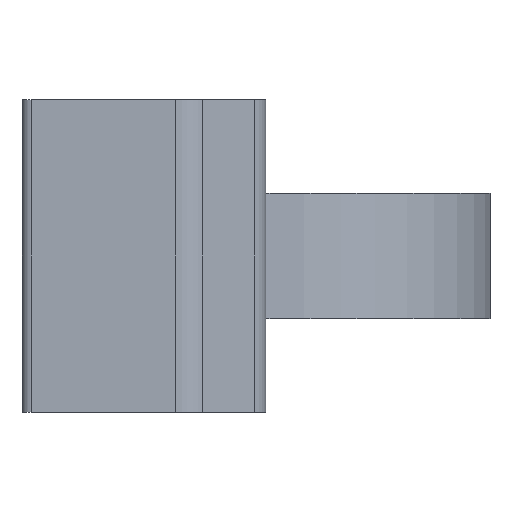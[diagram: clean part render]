
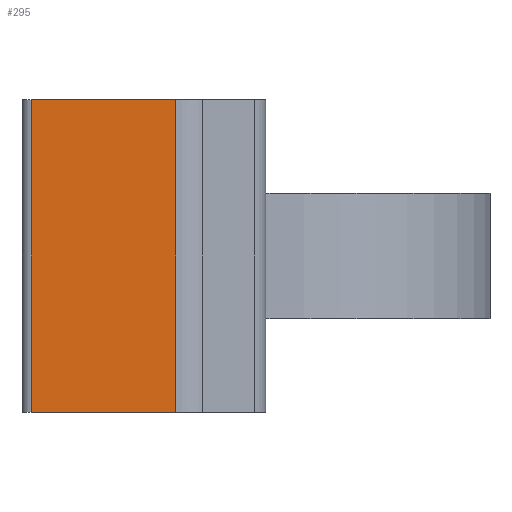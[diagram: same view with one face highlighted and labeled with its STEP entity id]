
A CAD part, front view. The second image highlights one B-rep face of the part: STEP entity #295.
In plain terms, the highlighted planar face has unit normal (0, -1, 0).
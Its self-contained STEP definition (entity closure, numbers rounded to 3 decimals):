
#17 = VECTOR ( 'NONE', #933, 1000. ) ;
#22 = ORIENTED_EDGE ( 'NONE', *, *, #569, .F. ) ;
#40 = VERTEX_POINT ( 'NONE', #56 ) ;
#45 = DIRECTION ( 'NONE',  ( 0., 1., 0. ) ) ;
#47 = VECTOR ( 'NONE', #1028, 1000. ) ;
#56 = CARTESIAN_POINT ( 'NONE',  ( 20.512, -13.319, -1.225 ) ) ;
#84 = ORIENTED_EDGE ( 'NONE', *, *, #685, .F. ) ;
#121 = CARTESIAN_POINT ( 'NONE',  ( 24.373, -13.319, -1.225 ) ) ;
#177 = EDGE_CURVE ( 'NONE', #637, #546, #1079, .T. ) ;
#223 = CARTESIAN_POINT ( 'NONE',  ( 23.524, -13.319, -1.225 ) ) ;
#237 = CARTESIAN_POINT ( 'NONE',  ( 24.373, -13.319, 7.125 ) ) ;
#295 = ADVANCED_FACE ( 'NONE', ( #660 ), #645, .F. ) ;
#318 = CARTESIAN_POINT ( 'NONE',  ( 20.512, -13.319, 2.95 ) ) ;
#405 = VERTEX_POINT ( 'NONE', #584 ) ;
#422 = DIRECTION ( 'NONE',  ( 0., 0., 1. ) ) ;
#431 = CARTESIAN_POINT ( 'NONE',  ( 23.524, -13.319, 7.125 ) ) ;
#469 = CARTESIAN_POINT ( 'NONE',  ( 24.373, -13.319, 2.95 ) ) ;
#546 = VERTEX_POINT ( 'NONE', #121 ) ;
#556 = LINE ( 'NONE', #431, #17 ) ;
#563 = EDGE_CURVE ( 'NONE', #40, #546, #643, .T. ) ;
#569 = EDGE_CURVE ( 'NONE', #405, #637, #556, .T. ) ;
#584 = CARTESIAN_POINT ( 'NONE',  ( 20.512, -13.319, 7.125 ) ) ;
#606 = ORIENTED_EDGE ( 'NONE', *, *, #563, .T. ) ;
#637 = VERTEX_POINT ( 'NONE', #237 ) ;
#643 = LINE ( 'NONE', #223, #47 ) ;
#645 = PLANE ( 'NONE',  #1106 ) ;
#655 = VECTOR ( 'NONE', #422, 1000. ) ;
#660 = FACE_OUTER_BOUND ( 'NONE', #1269, .T. ) ;
#685 = EDGE_CURVE ( 'NONE', #40, #405, #688, .T. ) ;
#688 = LINE ( 'NONE', #318, #655 ) ;
#753 = DIRECTION ( 'NONE',  ( 0., 0., 1. ) ) ;
#809 = VECTOR ( 'NONE', #967, 1000. ) ;
#814 = ORIENTED_EDGE ( 'NONE', *, *, #177, .F. ) ;
#933 = DIRECTION ( 'NONE',  ( 1., 0., 0. ) ) ;
#967 = DIRECTION ( 'NONE',  ( 0., 0., -1. ) ) ;
#1028 = DIRECTION ( 'NONE',  ( 1., 0., 0. ) ) ;
#1079 = LINE ( 'NONE', #469, #809 ) ;
#1106 = AXIS2_PLACEMENT_3D ( 'NONE', #1251, #45, #753 ) ;
#1251 = CARTESIAN_POINT ( 'NONE',  ( 20.512, -13.319, -1.225 ) ) ;
#1269 = EDGE_LOOP ( 'NONE', ( #606, #814, #22, #84 ) ) ;
